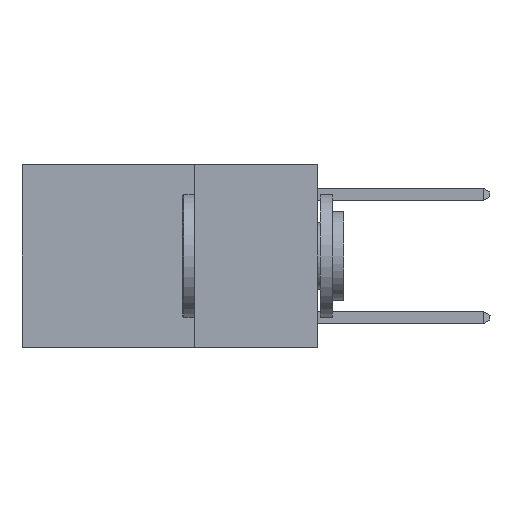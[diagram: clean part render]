
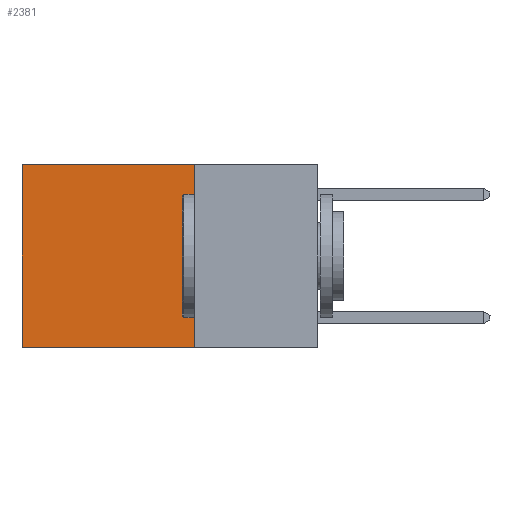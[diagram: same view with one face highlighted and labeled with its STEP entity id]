
A CAD part, left-side view. The second image highlights one B-rep face of the part: STEP entity #2381.
In plain terms, the highlighted planar face has unit normal (-1, 0, 0).
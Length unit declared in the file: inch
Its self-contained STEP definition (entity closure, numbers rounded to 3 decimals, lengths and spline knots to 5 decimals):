
#259 = AXIS2_PLACEMENT_3D ( 'NONE', #6963, #5189, #9314 ) ;
#319 = VECTOR ( 'NONE', #22952, 39.37008 ) ;
#2381 = ADVANCED_FACE ( 'NONE', ( #23925 ), #6829, .F. ) ;
#2831 = CARTESIAN_POINT ( 'NONE',  ( 0.2625, 0.25, 0. ) ) ;
#4139 = EDGE_CURVE ( 'NONE', #19211, #22703, #11198, .T. ) ;
#5189 = DIRECTION ( 'NONE',  ( 1., 0., 0. ) ) ;
#5888 = DIRECTION ( 'NONE',  ( 0., 0., -1. ) ) ;
#6278 = LINE ( 'NONE', #18768, #10447 ) ;
#6829 = PLANE ( 'NONE',  #259 ) ;
#6963 = CARTESIAN_POINT ( 'NONE',  ( 0.2625, 0.25, 0. ) ) ;
#9314 = DIRECTION ( 'NONE',  ( 0., 0., -1. ) ) ;
#10447 = VECTOR ( 'NONE', #5888, 39.37008 ) ;
#11198 = LINE ( 'NONE', #2831, #25316 ) ;
#12359 = ORIENTED_EDGE ( 'NONE', *, *, #22035, .T. ) ;
#12645 = EDGE_LOOP ( 'NONE', ( #12359, #16944, #26678, #23472 ) ) ;
#12855 = CARTESIAN_POINT ( 'NONE',  ( 0.2625, 0.25, 0. ) ) ;
#13146 = LINE ( 'NONE', #19832, #20436 ) ;
#13854 = CARTESIAN_POINT ( 'NONE',  ( 0.2625, 0.25, 0. ) ) ;
#14339 = EDGE_CURVE ( 'NONE', #19211, #20826, #23226, .T. ) ;
#16944 = ORIENTED_EDGE ( 'NONE', *, *, #19640, .F. ) ;
#18768 = CARTESIAN_POINT ( 'NONE',  ( 0.2625, 0.6, 0. ) ) ;
#19031 = CARTESIAN_POINT ( 'NONE',  ( 0.2625, 0.25, -0.37 ) ) ;
#19211 = VERTEX_POINT ( 'NONE', #13854 ) ;
#19640 = EDGE_CURVE ( 'NONE', #20826, #23583, #13146, .T. ) ;
#19701 = DIRECTION ( 'NONE',  ( 0., 1., 0. ) ) ;
#19832 = CARTESIAN_POINT ( 'NONE',  ( 0.2625, 0.25, -0.37 ) ) ;
#20102 = CARTESIAN_POINT ( 'NONE',  ( 0.2625, 0.6, -0.37 ) ) ;
#20436 = VECTOR ( 'NONE', #19701, 39.37008 ) ;
#20826 = VERTEX_POINT ( 'NONE', #19031 ) ;
#21846 = CARTESIAN_POINT ( 'NONE',  ( 0.2625, 0.6, 0. ) ) ;
#21990 = DIRECTION ( 'NONE',  ( 0., 1., 0. ) ) ;
#22035 = EDGE_CURVE ( 'NONE', #22703, #23583, #6278, .T. ) ;
#22703 = VERTEX_POINT ( 'NONE', #21846 ) ;
#22952 = DIRECTION ( 'NONE',  ( 0., 0., -1. ) ) ;
#23226 = LINE ( 'NONE', #12855, #319 ) ;
#23472 = ORIENTED_EDGE ( 'NONE', *, *, #4139, .T. ) ;
#23583 = VERTEX_POINT ( 'NONE', #20102 ) ;
#23925 = FACE_OUTER_BOUND ( 'NONE', #12645, .T. ) ;
#25316 = VECTOR ( 'NONE', #21990, 39.37008 ) ;
#26678 = ORIENTED_EDGE ( 'NONE', *, *, #14339, .F. ) ;
